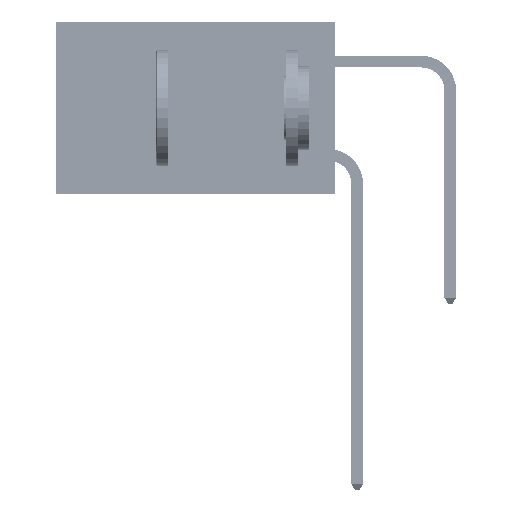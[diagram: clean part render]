
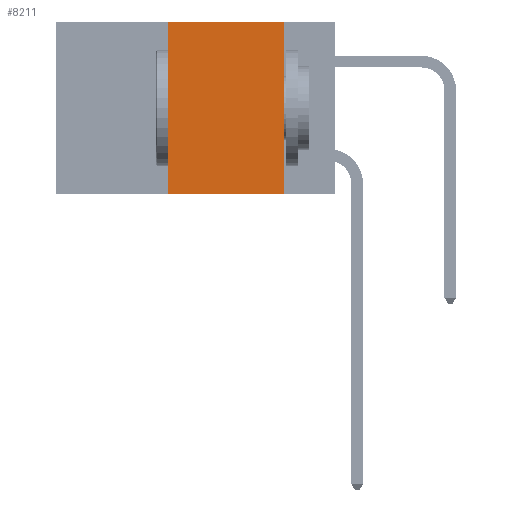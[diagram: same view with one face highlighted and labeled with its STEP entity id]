
A CAD part, left-side view. The second image highlights one B-rep face of the part: STEP entity #8211.
In plain terms, the highlighted planar face has unit normal (-1, 0, 0).
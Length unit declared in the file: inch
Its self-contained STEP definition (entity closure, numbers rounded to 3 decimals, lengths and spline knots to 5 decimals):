
#1411 = CARTESIAN_POINT ( 'NONE',  ( 0., 0.36, -0.37 ) ) ;
#1620 = CARTESIAN_POINT ( 'NONE',  ( 0., 0.36, 0. ) ) ;
#2108 = AXIS2_PLACEMENT_3D ( 'NONE', #23555, #41278, #12095 ) ;
#2528 = DIRECTION ( 'NONE',  ( 0., -1., 0. ) ) ;
#6732 = VERTEX_POINT ( 'NONE', #10704 ) ;
#8211 = ADVANCED_FACE ( 'NONE', ( #37038 ), #15960, .F. ) ;
#9674 = VECTOR ( 'NONE', #2528, 39.37008 ) ;
#10679 = LINE ( 'NONE', #40715, #24520 ) ;
#10704 = CARTESIAN_POINT ( 'NONE',  ( 0., 0.11, 0. ) ) ;
#12095 = DIRECTION ( 'NONE',  ( 0., 0., -1. ) ) ;
#15436 = LINE ( 'NONE', #23455, #41391 ) ;
#15939 = EDGE_CURVE ( 'NONE', #16499, #43427, #34375, .T. ) ;
#15960 = PLANE ( 'NONE',  #2108 ) ;
#16499 = VERTEX_POINT ( 'NONE', #1411 ) ;
#17225 = CARTESIAN_POINT ( 'NONE',  ( 0., 0.6, 0. ) ) ;
#18242 = CARTESIAN_POINT ( 'NONE',  ( 0., 0.11, -0.37 ) ) ;
#18304 = ORIENTED_EDGE ( 'NONE', *, *, #25521, .F. ) ;
#19456 = LINE ( 'NONE', #17225, #9674 ) ;
#19600 = DIRECTION ( 'NONE',  ( 0., 0., -1. ) ) ;
#21300 = EDGE_CURVE ( 'NONE', #16499, #29850, #15436, .T. ) ;
#23455 = CARTESIAN_POINT ( 'NONE',  ( 0., 0.6, -0.37 ) ) ;
#23555 = CARTESIAN_POINT ( 'NONE',  ( 0., 0.6, 0. ) ) ;
#24009 = EDGE_CURVE ( 'NONE', #43427, #6732, #19456, .T. ) ;
#24520 = VECTOR ( 'NONE', #19600, 39.37008 ) ;
#25521 = EDGE_CURVE ( 'NONE', #6732, #29850, #10679, .T. ) ;
#25532 = EDGE_LOOP ( 'NONE', ( #18304, #35227, #41427, #31205 ) ) ;
#29850 = VERTEX_POINT ( 'NONE', #18242 ) ;
#30694 = DIRECTION ( 'NONE',  ( 0., -1., 0. ) ) ;
#31205 = ORIENTED_EDGE ( 'NONE', *, *, #21300, .T. ) ;
#34375 = LINE ( 'NONE', #37607, #42556 ) ;
#35227 = ORIENTED_EDGE ( 'NONE', *, *, #24009, .F. ) ;
#37038 = FACE_OUTER_BOUND ( 'NONE', #25532, .T. ) ;
#37607 = CARTESIAN_POINT ( 'NONE',  ( 0., 0.36, 0. ) ) ;
#40715 = CARTESIAN_POINT ( 'NONE',  ( 0., 0.11, 0. ) ) ;
#41025 = DIRECTION ( 'NONE',  ( 0., 0., 1. ) ) ;
#41278 = DIRECTION ( 'NONE',  ( 1., 0., 0. ) ) ;
#41391 = VECTOR ( 'NONE', #30694, 39.37008 ) ;
#41427 = ORIENTED_EDGE ( 'NONE', *, *, #15939, .F. ) ;
#42556 = VECTOR ( 'NONE', #41025, 39.37008 ) ;
#43427 = VERTEX_POINT ( 'NONE', #1620 ) ;
